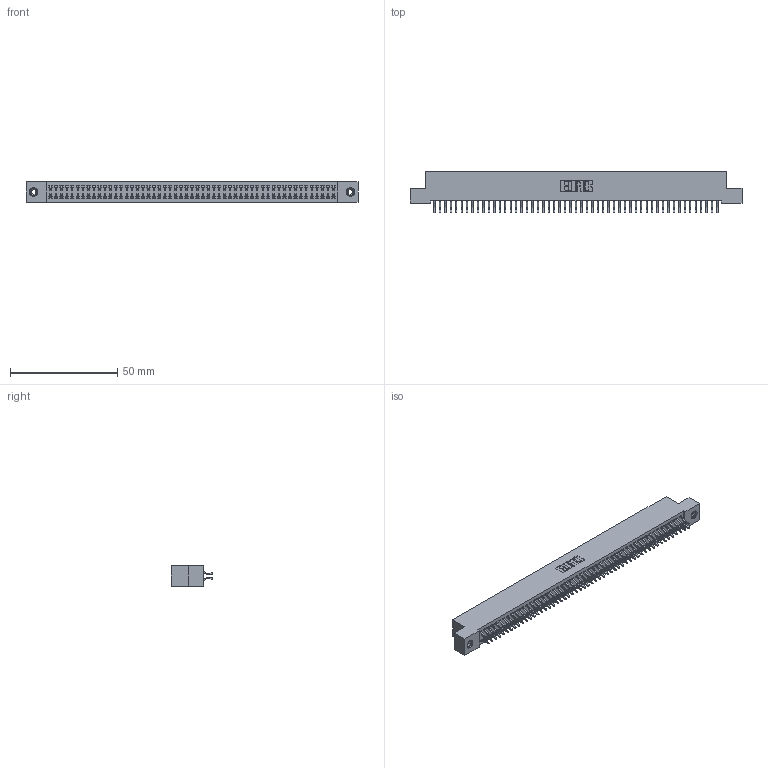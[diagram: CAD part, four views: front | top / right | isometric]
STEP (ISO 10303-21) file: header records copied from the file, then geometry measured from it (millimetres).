
FILE_DESCRIPTION (( 'STEP AP203' ), '1' );
FILE_NAME ('342-106-556-208.STEP', '2018-08-14T07:14:53', ( '' ), ( '' ), 'SwSTEP 2.0', 'SolidWorks 2016', '' );
FILE_SCHEMA (( 'CONFIG_CONTROL_DESIGN' ));
Length unit declared in the file: inch
Products named in the file (4): 342 Part_TI; 345-292-001_556 Tail; 345-250-001_345-250-003-102; 342-106-556-208
Assembly tree (109 placements, depth 2):
  342-106-556-208
    342 Part_TI
    345-292-001_556 Tail  x106
    345-250-001_345-250-003-102  x2
Bounding box: 154.94 x 19.58 x 9.4 mm (x, y, z)
Volume: 13965 mm3; surface area: 22910.1 mm2
Topology: 109 solids, 109 shells, 6318 faces, 18773 edges, 12366 vertices
Faces by surface type: plane 4338, cylinder 1964, cone 12, torus 4
Entity records: 33948 total; most frequent: CARTESIAN_POINT 5609, ORIENTED_EDGE 5526, DIRECTION 4793, EDGE_CURVE 2763, LINE 2607, VECTOR 2607, VERTEX_POINT 1836, AXIS2_PLACEMENT_3D 1093
